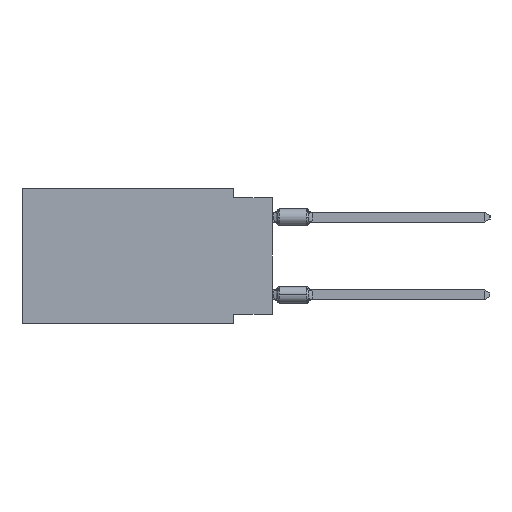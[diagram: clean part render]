
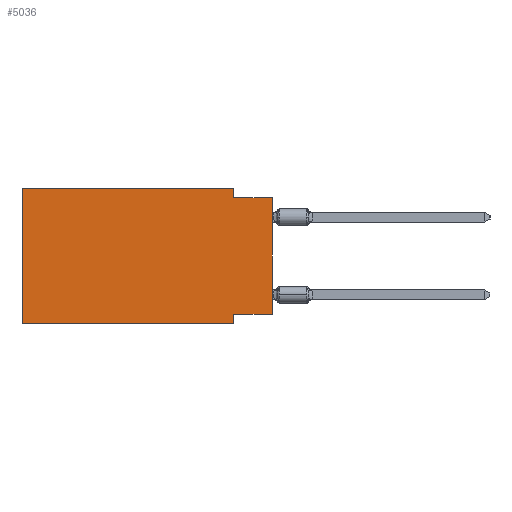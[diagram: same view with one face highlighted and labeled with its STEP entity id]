
A CAD part, left-side view. The second image highlights one B-rep face of the part: STEP entity #5036.
In plain terms, the highlighted planar face has unit normal (-1, 0, 0).
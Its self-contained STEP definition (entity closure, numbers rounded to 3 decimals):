
#120 = ORIENTED_EDGE ( 'NONE', *, *, #22402, .F. ) ;
#615 = LINE ( 'NONE', #21869, #8302 ) ;
#1201 = DIRECTION ( 'NONE',  ( 0., -1., 0. ) ) ;
#2023 = VERTEX_POINT ( 'NONE', #19648 ) ;
#3431 = LINE ( 'NONE', #8448, #15453 ) ;
#3458 = DIRECTION ( 'NONE',  ( 0., -1., 0. ) ) ;
#3888 = LINE ( 'NONE', #19792, #9021 ) ;
#4104 = CARTESIAN_POINT ( 'NONE',  ( 0., 2.54, 0. ) ) ;
#4755 = EDGE_CURVE ( 'NONE', #8715, #9980, #14369, .T. ) ;
#5036 = ADVANCED_FACE ( 'NONE', ( #9097 ), #30698, .F. ) ;
#5950 = VECTOR ( 'NONE', #15810, 1000. ) ;
#6216 = CARTESIAN_POINT ( 'NONE',  ( 0., 0., -0.635 ) ) ;
#7131 = ORIENTED_EDGE ( 'NONE', *, *, #4755, .F. ) ;
#8006 = CARTESIAN_POINT ( 'NONE',  ( 0., 16.383, -8.89 ) ) ;
#8302 = VECTOR ( 'NONE', #16375, 1000. ) ;
#8448 = CARTESIAN_POINT ( 'NONE',  ( 0., 0., 0. ) ) ;
#8715 = VERTEX_POINT ( 'NONE', #10677 ) ;
#9021 = VECTOR ( 'NONE', #32897, 1000. ) ;
#9081 = VERTEX_POINT ( 'NONE', #28979 ) ;
#9097 = FACE_OUTER_BOUND ( 'NONE', #19551, .T. ) ;
#9675 = VERTEX_POINT ( 'NONE', #20041 ) ;
#9915 = DIRECTION ( 'NONE',  ( 0., 1., 0. ) ) ;
#9980 = VERTEX_POINT ( 'NONE', #4104 ) ;
#10677 = CARTESIAN_POINT ( 'NONE',  ( 0., 16.383, 0. ) ) ;
#11073 = CARTESIAN_POINT ( 'NONE',  ( 0., 16.383, 0. ) ) ;
#12790 = EDGE_CURVE ( 'NONE', #33356, #9675, #17234, .T. ) ;
#14369 = LINE ( 'NONE', #11073, #27447 ) ;
#15297 = CARTESIAN_POINT ( 'NONE',  ( 0., 2.54, -8.255 ) ) ;
#15453 = VECTOR ( 'NONE', #19348, 1000. ) ;
#15810 = DIRECTION ( 'NONE',  ( 0., 0., -1. ) ) ;
#16070 = CARTESIAN_POINT ( 'NONE',  ( 0., 0., -0.635 ) ) ;
#16145 = VECTOR ( 'NONE', #22060, 1000. ) ;
#16375 = DIRECTION ( 'NONE',  ( 0., -1., 0. ) ) ;
#17230 = ORIENTED_EDGE ( 'NONE', *, *, #27292, .T. ) ;
#17234 = LINE ( 'NONE', #24682, #16145 ) ;
#17529 = AXIS2_PLACEMENT_3D ( 'NONE', #22417, #27770, #19657 ) ;
#18504 = EDGE_CURVE ( 'NONE', #22447, #8715, #3888, .T. ) ;
#18905 = CARTESIAN_POINT ( 'NONE',  ( 0., 2.54, 0. ) ) ;
#19288 = EDGE_CURVE ( 'NONE', #2023, #28753, #22805, .T. ) ;
#19348 = DIRECTION ( 'NONE',  ( 0., 0., 1. ) ) ;
#19551 = EDGE_LOOP ( 'NONE', ( #28017, #32937, #29487, #7131, #34164, #17230, #25878, #120 ) ) ;
#19648 = CARTESIAN_POINT ( 'NONE',  ( 0., 2.54, -0.635 ) ) ;
#19657 = DIRECTION ( 'NONE',  ( 0., 0., -1. ) ) ;
#19792 = CARTESIAN_POINT ( 'NONE',  ( 0., 16.383, 0. ) ) ;
#20041 = CARTESIAN_POINT ( 'NONE',  ( 0., 2.54, -8.89 ) ) ;
#21869 = CARTESIAN_POINT ( 'NONE',  ( 0., 16.383, -8.89 ) ) ;
#22060 = DIRECTION ( 'NONE',  ( 0., 0., -1. ) ) ;
#22336 = VECTOR ( 'NONE', #1201, 1000. ) ;
#22402 = EDGE_CURVE ( 'NONE', #9081, #33356, #30833, .T. ) ;
#22414 = EDGE_CURVE ( 'NONE', #9980, #2023, #24087, .T. ) ;
#22417 = CARTESIAN_POINT ( 'NONE',  ( 0., 16.383, 0. ) ) ;
#22447 = VERTEX_POINT ( 'NONE', #8006 ) ;
#22805 = LINE ( 'NONE', #6216, #22336 ) ;
#24087 = LINE ( 'NONE', #18905, #5950 ) ;
#24682 = CARTESIAN_POINT ( 'NONE',  ( 0., 2.54, -8.89 ) ) ;
#25878 = ORIENTED_EDGE ( 'NONE', *, *, #12790, .F. ) ;
#27292 = EDGE_CURVE ( 'NONE', #22447, #9675, #615, .T. ) ;
#27447 = VECTOR ( 'NONE', #3458, 1000. ) ;
#27770 = DIRECTION ( 'NONE',  ( 1., 0., 0. ) ) ;
#28017 = ORIENTED_EDGE ( 'NONE', *, *, #30132, .T. ) ;
#28753 = VERTEX_POINT ( 'NONE', #16070 ) ;
#28979 = CARTESIAN_POINT ( 'NONE',  ( 0., 0., -8.255 ) ) ;
#29487 = ORIENTED_EDGE ( 'NONE', *, *, #22414, .F. ) ;
#30132 = EDGE_CURVE ( 'NONE', #9081, #28753, #3431, .T. ) ;
#30698 = PLANE ( 'NONE',  #17529 ) ;
#30833 = LINE ( 'NONE', #33578, #31333 ) ;
#31333 = VECTOR ( 'NONE', #9915, 1000. ) ;
#32897 = DIRECTION ( 'NONE',  ( 0., 0., 1. ) ) ;
#32937 = ORIENTED_EDGE ( 'NONE', *, *, #19288, .F. ) ;
#33356 = VERTEX_POINT ( 'NONE', #15297 ) ;
#33578 = CARTESIAN_POINT ( 'NONE',  ( 0., 0., -8.255 ) ) ;
#34164 = ORIENTED_EDGE ( 'NONE', *, *, #18504, .F. ) ;
